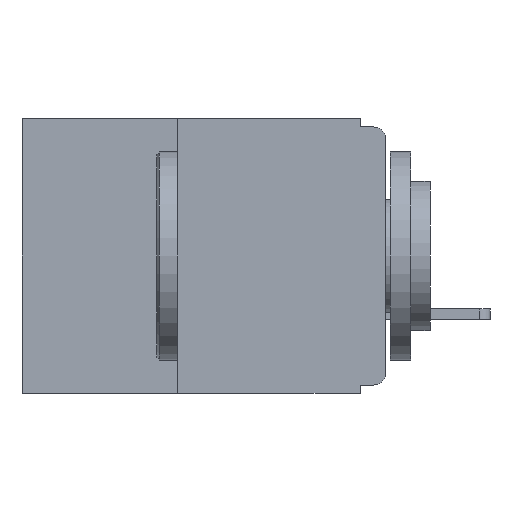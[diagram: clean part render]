
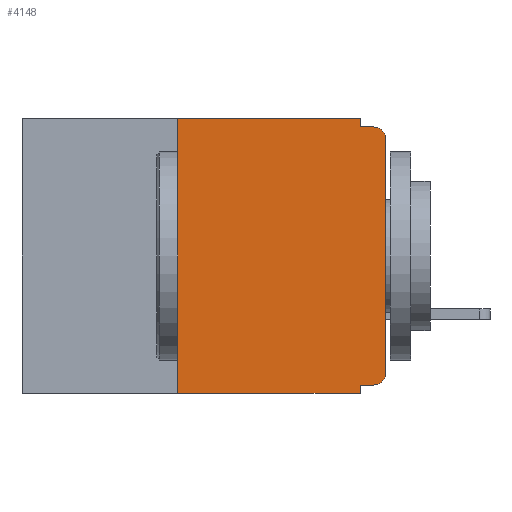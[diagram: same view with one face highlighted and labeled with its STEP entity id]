
A CAD part, left-side view. The second image highlights one B-rep face of the part: STEP entity #4148.
In plain terms, the highlighted planar face has unit normal (-1, 0, 0).
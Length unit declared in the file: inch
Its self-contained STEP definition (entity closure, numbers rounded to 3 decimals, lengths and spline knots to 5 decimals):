
#204 = VERTEX_POINT ( 'NONE', #3022 ) ;
#270 = VECTOR ( 'NONE', #22812, 39.37008 ) ;
#320 = VECTOR ( 'NONE', #12987, 39.37008 ) ;
#512 = DIRECTION ( 'NONE',  ( -1., 0., 0. ) ) ;
#909 = FACE_OUTER_BOUND ( 'NONE', #8294, .T. ) ;
#1050 = VERTEX_POINT ( 'NONE', #20530 ) ;
#1245 = CARTESIAN_POINT ( 'NONE',  ( 0., 0.437, -0.33 ) ) ;
#1652 = CARTESIAN_POINT ( 'NONE',  ( 0., 0.015, -0.305 ) ) ;
#1673 = VECTOR ( 'NONE', #6963, 39.37008 ) ;
#1826 = CARTESIAN_POINT ( 'NONE',  ( 0., 0.25, -0.33 ) ) ;
#2030 = CIRCLE ( 'NONE', #11181, 0.015 ) ;
#2637 = VERTEX_POINT ( 'NONE', #7119 ) ;
#3022 = CARTESIAN_POINT ( 'NONE',  ( 0., 0.031, 0. ) ) ;
#3072 = DIRECTION ( 'NONE',  ( 0., -1., 0. ) ) ;
#3505 = DIRECTION ( 'NONE',  ( 0., 0., -1. ) ) ;
#3805 = ORIENTED_EDGE ( 'NONE', *, *, #6591, .F. ) ;
#3971 = CARTESIAN_POINT ( 'NONE',  ( 0., 0.031, -0.32 ) ) ;
#4136 = VECTOR ( 'NONE', #9586, 39.37008 ) ;
#4148 = ADVANCED_FACE ( 'NONE', ( #909 ), #6538, .F. ) ;
#5166 = LINE ( 'NONE', #9388, #320 ) ;
#5582 = VERTEX_POINT ( 'NONE', #1826 ) ;
#6046 = EDGE_CURVE ( 'NONE', #12084, #1050, #11293, .T. ) ;
#6095 = DIRECTION ( 'NONE',  ( 0., 1., 0. ) ) ;
#6105 = ORIENTED_EDGE ( 'NONE', *, *, #19927, .F. ) ;
#6316 = DIRECTION ( 'NONE',  ( 0., 0., -1. ) ) ;
#6422 = DIRECTION ( 'NONE',  ( 1., 0., 0. ) ) ;
#6538 = PLANE ( 'NONE',  #12706 ) ;
#6543 = CARTESIAN_POINT ( 'NONE',  ( 0., 0.031, 0. ) ) ;
#6591 = EDGE_CURVE ( 'NONE', #204, #8760, #19483, .T. ) ;
#6963 = DIRECTION ( 'NONE',  ( 0., 0., -1. ) ) ;
#7119 = CARTESIAN_POINT ( 'NONE',  ( 0., 0.015, -0.32 ) ) ;
#7623 = EDGE_CURVE ( 'NONE', #15928, #8913, #7909, .T. ) ;
#7659 = CARTESIAN_POINT ( 'NONE',  ( 0., 0.437, 0. ) ) ;
#7909 = CIRCLE ( 'NONE', #10956, 0.015 ) ;
#8294 = EDGE_LOOP ( 'NONE', ( #16914, #22091, #11648, #3805, #6105, #15152, #11439, #14946, #14735, #20281 ) ) ;
#8760 = VERTEX_POINT ( 'NONE', #13134 ) ;
#8913 = VERTEX_POINT ( 'NONE', #17129 ) ;
#9192 = CARTESIAN_POINT ( 'NONE',  ( 0., 0.25, -0.33 ) ) ;
#9295 = EDGE_CURVE ( 'NONE', #9360, #15928, #18499, .T. ) ;
#9360 = VERTEX_POINT ( 'NONE', #20593 ) ;
#9388 = CARTESIAN_POINT ( 'NONE',  ( 0., 0., -0.01 ) ) ;
#9586 = DIRECTION ( 'NONE',  ( 0., 0., 1. ) ) ;
#9717 = VECTOR ( 'NONE', #3072, 39.37008 ) ;
#9761 = CARTESIAN_POINT ( 'NONE',  ( 0., 0., -0.025 ) ) ;
#10005 = LINE ( 'NONE', #20257, #20156 ) ;
#10956 = AXIS2_PLACEMENT_3D ( 'NONE', #11347, #512, #13168 ) ;
#11181 = AXIS2_PLACEMENT_3D ( 'NONE', #1652, #14292, #3505 ) ;
#11293 = LINE ( 'NONE', #23221, #1673 ) ;
#11347 = CARTESIAN_POINT ( 'NONE',  ( 0., 0.015, -0.025 ) ) ;
#11439 = ORIENTED_EDGE ( 'NONE', *, *, #20824, .T. ) ;
#11648 = ORIENTED_EDGE ( 'NONE', *, *, #21454, .F. ) ;
#11995 = EDGE_CURVE ( 'NONE', #5582, #13799, #12434, .T. ) ;
#12084 = VERTEX_POINT ( 'NONE', #3971 ) ;
#12434 = LINE ( 'NONE', #9192, #13010 ) ;
#12706 = AXIS2_PLACEMENT_3D ( 'NONE', #7659, #6422, #6316 ) ;
#12987 = DIRECTION ( 'NONE',  ( 0., -1., 0. ) ) ;
#13010 = VECTOR ( 'NONE', #19976, 39.37008 ) ;
#13134 = CARTESIAN_POINT ( 'NONE',  ( 0., 0.031, -0.01 ) ) ;
#13168 = DIRECTION ( 'NONE',  ( 0., 0., -1. ) ) ;
#13674 = EDGE_CURVE ( 'NONE', #2637, #9360, #2030, .T. ) ;
#13799 = VERTEX_POINT ( 'NONE', #18229 ) ;
#14292 = DIRECTION ( 'NONE',  ( -1., 0., 0. ) ) ;
#14735 = ORIENTED_EDGE ( 'NONE', *, *, #19309, .F. ) ;
#14789 = DIRECTION ( 'NONE',  ( 0., -1., 0. ) ) ;
#14946 = ORIENTED_EDGE ( 'NONE', *, *, #6046, .F. ) ;
#15152 = ORIENTED_EDGE ( 'NONE', *, *, #11995, .F. ) ;
#15928 = VERTEX_POINT ( 'NONE', #9761 ) ;
#16156 = VECTOR ( 'NONE', #6095, 39.37008 ) ;
#16914 = ORIENTED_EDGE ( 'NONE', *, *, #9295, .T. ) ;
#17129 = CARTESIAN_POINT ( 'NONE',  ( 0., 0.015, -0.01 ) ) ;
#18229 = CARTESIAN_POINT ( 'NONE',  ( 0., 0.25, 0. ) ) ;
#18499 = LINE ( 'NONE', #18541, #4136 ) ;
#18541 = CARTESIAN_POINT ( 'NONE',  ( 0., 0., 0. ) ) ;
#19290 = LINE ( 'NONE', #1245, #9717 ) ;
#19309 = EDGE_CURVE ( 'NONE', #2637, #12084, #20414, .T. ) ;
#19483 = LINE ( 'NONE', #6543, #270 ) ;
#19927 = EDGE_CURVE ( 'NONE', #13799, #204, #10005, .T. ) ;
#19976 = DIRECTION ( 'NONE',  ( 0., 0., 1. ) ) ;
#20156 = VECTOR ( 'NONE', #14789, 39.37008 ) ;
#20257 = CARTESIAN_POINT ( 'NONE',  ( 0., 0.437, 0. ) ) ;
#20281 = ORIENTED_EDGE ( 'NONE', *, *, #13674, .T. ) ;
#20414 = LINE ( 'NONE', #20511, #16156 ) ;
#20511 = CARTESIAN_POINT ( 'NONE',  ( 0., 0., -0.32 ) ) ;
#20530 = CARTESIAN_POINT ( 'NONE',  ( 0., 0.031, -0.33 ) ) ;
#20593 = CARTESIAN_POINT ( 'NONE',  ( 0., 0., -0.305 ) ) ;
#20824 = EDGE_CURVE ( 'NONE', #5582, #1050, #19290, .T. ) ;
#21454 = EDGE_CURVE ( 'NONE', #8760, #8913, #5166, .T. ) ;
#22091 = ORIENTED_EDGE ( 'NONE', *, *, #7623, .T. ) ;
#22812 = DIRECTION ( 'NONE',  ( 0., 0., -1. ) ) ;
#23221 = CARTESIAN_POINT ( 'NONE',  ( 0., 0.031, -0.33 ) ) ;
